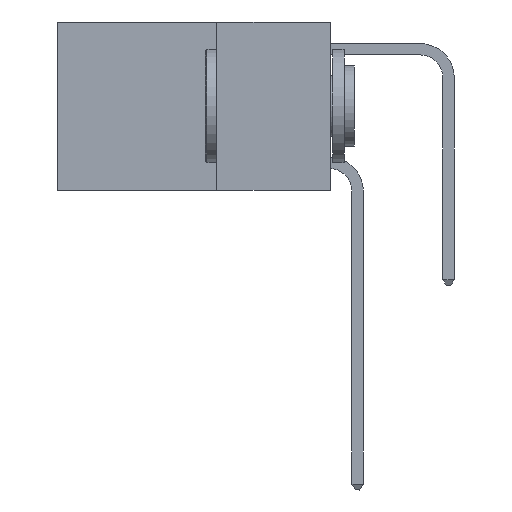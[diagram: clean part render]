
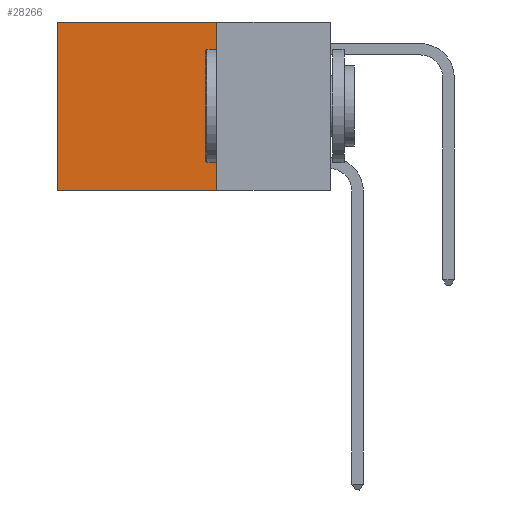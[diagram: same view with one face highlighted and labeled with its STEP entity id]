
A CAD part, left-side view. The second image highlights one B-rep face of the part: STEP entity #28266.
In plain terms, the highlighted planar face has unit normal (-1, 0, 0).
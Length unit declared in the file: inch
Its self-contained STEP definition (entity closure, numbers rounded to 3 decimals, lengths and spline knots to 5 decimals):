
#81 = CARTESIAN_POINT ( 'NONE',  ( 0.2625, 0.25, 0. ) ) ;
#1537 = EDGE_LOOP ( 'NONE', ( #3291, #11970, #12954, #20644 ) ) ;
#3291 = ORIENTED_EDGE ( 'NONE', *, *, #5045, .T. ) ;
#3793 = CARTESIAN_POINT ( 'NONE',  ( 0.2625, 0.25, -0.37 ) ) ;
#4209 = EDGE_CURVE ( 'NONE', #11773, #23381, #10487, .T. ) ;
#4473 = CARTESIAN_POINT ( 'NONE',  ( 0.2625, 0.25, 0. ) ) ;
#4602 = LINE ( 'NONE', #81, #23972 ) ;
#5041 = AXIS2_PLACEMENT_3D ( 'NONE', #18897, #25579, #16868 ) ;
#5045 = EDGE_CURVE ( 'NONE', #18620, #23381, #11419, .T. ) ;
#5459 = CARTESIAN_POINT ( 'NONE',  ( 0.2625, 0.25, -0.37 ) ) ;
#7175 = EDGE_CURVE ( 'NONE', #14813, #11773, #26075, .T. ) ;
#10017 = FACE_OUTER_BOUND ( 'NONE', #1537, .T. ) ;
#10487 = LINE ( 'NONE', #3793, #16930 ) ;
#11035 = DIRECTION ( 'NONE',  ( 0., 1., 0. ) ) ;
#11419 = LINE ( 'NONE', #13755, #13680 ) ;
#11773 = VERTEX_POINT ( 'NONE', #5459 ) ;
#11970 = ORIENTED_EDGE ( 'NONE', *, *, #4209, .F. ) ;
#12954 = ORIENTED_EDGE ( 'NONE', *, *, #7175, .F. ) ;
#13680 = VECTOR ( 'NONE', #20298, 39.37008 ) ;
#13755 = CARTESIAN_POINT ( 'NONE',  ( 0.2625, 0.6, 0. ) ) ;
#14813 = VERTEX_POINT ( 'NONE', #4473 ) ;
#15037 = CARTESIAN_POINT ( 'NONE',  ( 0.2625, 0.25, 0. ) ) ;
#16868 = DIRECTION ( 'NONE',  ( 0., 0., -1. ) ) ;
#16930 = VECTOR ( 'NONE', #25752, 39.37008 ) ;
#17167 = PLANE ( 'NONE',  #5041 ) ;
#17980 = VECTOR ( 'NONE', #23885, 39.37008 ) ;
#18620 = VERTEX_POINT ( 'NONE', #28077 ) ;
#18897 = CARTESIAN_POINT ( 'NONE',  ( 0.2625, 0.25, 0. ) ) ;
#20298 = DIRECTION ( 'NONE',  ( 0., 0., -1. ) ) ;
#20372 = EDGE_CURVE ( 'NONE', #14813, #18620, #4602, .T. ) ;
#20644 = ORIENTED_EDGE ( 'NONE', *, *, #20372, .T. ) ;
#23381 = VERTEX_POINT ( 'NONE', #28267 ) ;
#23885 = DIRECTION ( 'NONE',  ( 0., 0., -1. ) ) ;
#23972 = VECTOR ( 'NONE', #11035, 39.37008 ) ;
#25579 = DIRECTION ( 'NONE',  ( 1., 0., 0. ) ) ;
#25752 = DIRECTION ( 'NONE',  ( 0., 1., 0. ) ) ;
#26075 = LINE ( 'NONE', #15037, #17980 ) ;
#28077 = CARTESIAN_POINT ( 'NONE',  ( 0.2625, 0.6, 0. ) ) ;
#28266 = ADVANCED_FACE ( 'NONE', ( #10017 ), #17167, .F. ) ;
#28267 = CARTESIAN_POINT ( 'NONE',  ( 0.2625, 0.6, -0.37 ) ) ;
